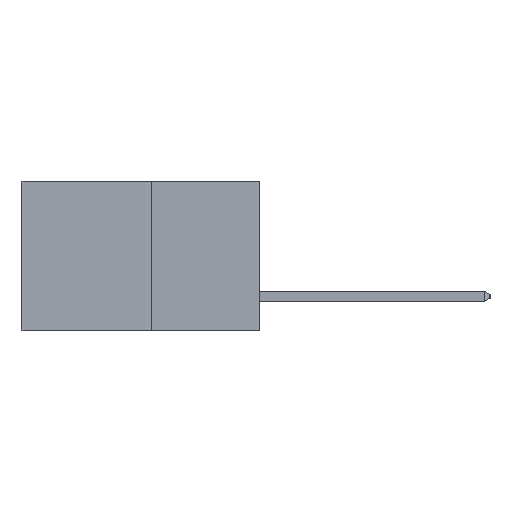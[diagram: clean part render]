
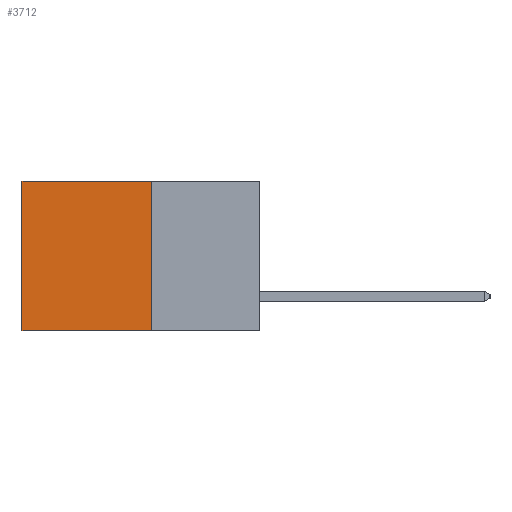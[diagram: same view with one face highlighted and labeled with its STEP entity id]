
A CAD part, left-side view. The second image highlights one B-rep face of the part: STEP entity #3712.
In plain terms, the highlighted planar face has unit normal (-1, 0, 0).
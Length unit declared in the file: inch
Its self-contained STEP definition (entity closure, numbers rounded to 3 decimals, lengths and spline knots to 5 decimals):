
#166 = EDGE_LOOP ( 'NONE', ( #1396, #390, #1078, #875 ) ) ;
#203 = AXIS2_PLACEMENT_3D ( 'NONE', #10435, #1165, #12795 ) ;
#390 = ORIENTED_EDGE ( 'NONE', *, *, #1485, .F. ) ;
#875 = ORIENTED_EDGE ( 'NONE', *, *, #5616, .T. ) ;
#890 = LINE ( 'NONE', #12020, #12552 ) ;
#1078 = ORIENTED_EDGE ( 'NONE', *, *, #10794, .F. ) ;
#1165 = DIRECTION ( 'NONE',  ( 1., 0., 0. ) ) ;
#1306 = VECTOR ( 'NONE', #11709, 39.37008 ) ;
#1396 = ORIENTED_EDGE ( 'NONE', *, *, #3371, .T. ) ;
#1485 = EDGE_CURVE ( 'NONE', #12500, #12043, #10373, .T. ) ;
#1670 = VERTEX_POINT ( 'NONE', #2487 ) ;
#1674 = PLANE ( 'NONE',  #203 ) ;
#1954 = DIRECTION ( 'NONE',  ( 0., 0., -1. ) ) ;
#2270 = CARTESIAN_POINT ( 'NONE',  ( 0.277, 0.59, -0.37 ) ) ;
#2487 = CARTESIAN_POINT ( 'NONE',  ( 0.277, 0.27, 0. ) ) ;
#3371 = EDGE_CURVE ( 'NONE', #8528, #12043, #12951, .T. ) ;
#3712 = ADVANCED_FACE ( 'NONE', ( #6260 ), #1674, .F. ) ;
#4439 = DIRECTION ( 'NONE',  ( 0., 0., -1. ) ) ;
#4781 = CARTESIAN_POINT ( 'NONE',  ( 0.277, 0.27, -0.37 ) ) ;
#5616 = EDGE_CURVE ( 'NONE', #1670, #8528, #890, .T. ) ;
#6260 = FACE_OUTER_BOUND ( 'NONE', #166, .T. ) ;
#8528 = VERTEX_POINT ( 'NONE', #12944 ) ;
#8758 = CARTESIAN_POINT ( 'NONE',  ( 0.277, 0.59, -0.37 ) ) ;
#8960 = VECTOR ( 'NONE', #1954, 39.37008 ) ;
#9684 = LINE ( 'NONE', #13091, #8960 ) ;
#10094 = VECTOR ( 'NONE', #4439, 39.37008 ) ;
#10373 = LINE ( 'NONE', #4781, #1306 ) ;
#10435 = CARTESIAN_POINT ( 'NONE',  ( 0.277, 0.27, -0.37 ) ) ;
#10794 = EDGE_CURVE ( 'NONE', #1670, #12500, #9684, .T. ) ;
#11161 = CARTESIAN_POINT ( 'NONE',  ( 0.277, 0.27, -0.37 ) ) ;
#11709 = DIRECTION ( 'NONE',  ( 0., 1., 0. ) ) ;
#11776 = DIRECTION ( 'NONE',  ( 0., 1., 0. ) ) ;
#12020 = CARTESIAN_POINT ( 'NONE',  ( 0.277, 0.27, 0. ) ) ;
#12043 = VERTEX_POINT ( 'NONE', #8758 ) ;
#12500 = VERTEX_POINT ( 'NONE', #11161 ) ;
#12552 = VECTOR ( 'NONE', #11776, 39.37008 ) ;
#12795 = DIRECTION ( 'NONE',  ( 0., 0., -1. ) ) ;
#12944 = CARTESIAN_POINT ( 'NONE',  ( 0.277, 0.59, 0. ) ) ;
#12951 = LINE ( 'NONE', #2270, #10094 ) ;
#13091 = CARTESIAN_POINT ( 'NONE',  ( 0.277, 0.27, -0.37 ) ) ;
